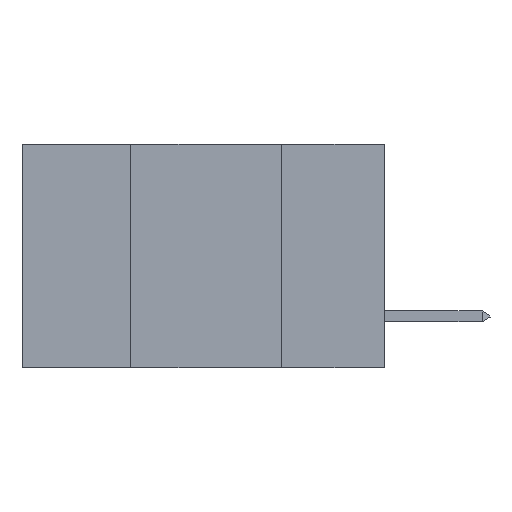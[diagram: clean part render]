
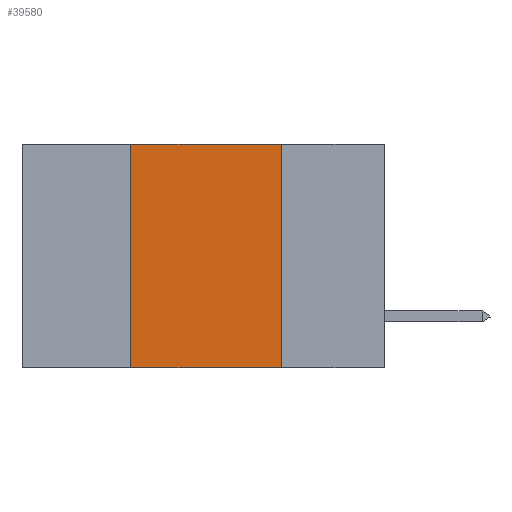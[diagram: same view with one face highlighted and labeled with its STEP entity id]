
A CAD part, left-side view. The second image highlights one B-rep face of the part: STEP entity #39580.
In plain terms, the highlighted planar face has unit normal (-1, 0, 0).
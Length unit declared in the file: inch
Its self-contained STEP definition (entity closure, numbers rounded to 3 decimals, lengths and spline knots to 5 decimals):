
#761 = CARTESIAN_POINT ( 'NONE',  ( 0., 0.42, -0.37 ) ) ;
#1342 = LINE ( 'NONE', #18479, #42992 ) ;
#1602 = VERTEX_POINT ( 'NONE', #761 ) ;
#3165 = LINE ( 'NONE', #38800, #13293 ) ;
#3924 = FACE_OUTER_BOUND ( 'NONE', #4600, .T. ) ;
#4531 = DIRECTION ( 'NONE',  ( 0., -1., 0. ) ) ;
#4600 = EDGE_LOOP ( 'NONE', ( #45904, #29591, #10632, #31217 ) ) ;
#4909 = DIRECTION ( 'NONE',  ( 0., -1., 0. ) ) ;
#10632 = ORIENTED_EDGE ( 'NONE', *, *, #25582, .F. ) ;
#11380 = DIRECTION ( 'NONE',  ( 0., 0., -1. ) ) ;
#12885 = CARTESIAN_POINT ( 'NONE',  ( 0., 0.6, 0. ) ) ;
#13293 = VECTOR ( 'NONE', #35487, 39.37008 ) ;
#14544 = EDGE_CURVE ( 'NONE', #21441, #22482, #1342, .T. ) ;
#15221 = CARTESIAN_POINT ( 'NONE',  ( 0., 0.42, 0. ) ) ;
#16658 = EDGE_CURVE ( 'NONE', #30856, #21441, #31528, .T. ) ;
#16787 = VECTOR ( 'NONE', #4909, 39.37008 ) ;
#18479 = CARTESIAN_POINT ( 'NONE',  ( 0., 0.17, 0. ) ) ;
#21441 = VERTEX_POINT ( 'NONE', #43614 ) ;
#22482 = VERTEX_POINT ( 'NONE', #31448 ) ;
#25582 = EDGE_CURVE ( 'NONE', #1602, #30856, #3165, .T. ) ;
#27557 = PLANE ( 'NONE',  #38107 ) ;
#29591 = ORIENTED_EDGE ( 'NONE', *, *, #16658, .F. ) ;
#30856 = VERTEX_POINT ( 'NONE', #15221 ) ;
#31148 = DIRECTION ( 'NONE',  ( 1., 0., 0. ) ) ;
#31217 = ORIENTED_EDGE ( 'NONE', *, *, #35812, .T. ) ;
#31448 = CARTESIAN_POINT ( 'NONE',  ( 0., 0.17, -0.37 ) ) ;
#31528 = LINE ( 'NONE', #44781, #41055 ) ;
#33576 = CARTESIAN_POINT ( 'NONE',  ( 0., 0.6, -0.37 ) ) ;
#35487 = DIRECTION ( 'NONE',  ( 0., 0., 1. ) ) ;
#35812 = EDGE_CURVE ( 'NONE', #1602, #22482, #39826, .T. ) ;
#38107 = AXIS2_PLACEMENT_3D ( 'NONE', #12885, #31148, #45599 ) ;
#38800 = CARTESIAN_POINT ( 'NONE',  ( 0., 0.42, 0. ) ) ;
#39580 = ADVANCED_FACE ( 'NONE', ( #3924 ), #27557, .F. ) ;
#39826 = LINE ( 'NONE', #33576, #16787 ) ;
#41055 = VECTOR ( 'NONE', #4531, 39.37008 ) ;
#42992 = VECTOR ( 'NONE', #11380, 39.37008 ) ;
#43614 = CARTESIAN_POINT ( 'NONE',  ( 0., 0.17, 0. ) ) ;
#44781 = CARTESIAN_POINT ( 'NONE',  ( 0., 0.6, 0. ) ) ;
#45599 = DIRECTION ( 'NONE',  ( 0., 0., -1. ) ) ;
#45904 = ORIENTED_EDGE ( 'NONE', *, *, #14544, .F. ) ;
